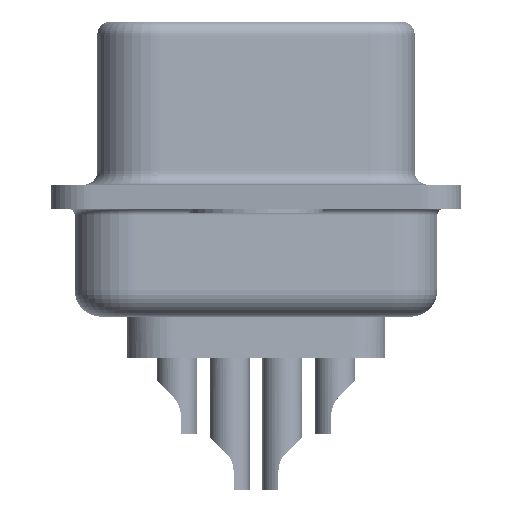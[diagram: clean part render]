
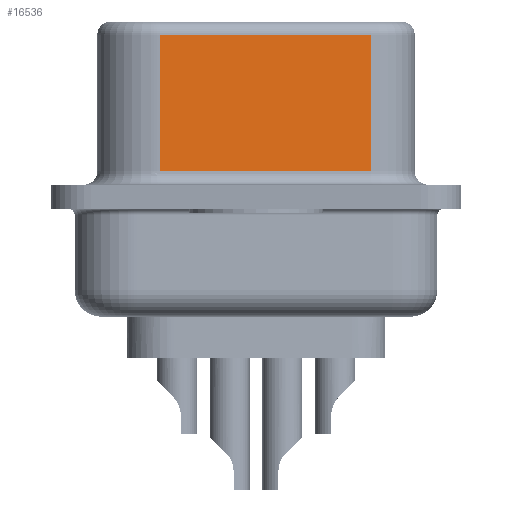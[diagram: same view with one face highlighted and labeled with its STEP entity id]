
A CAD part, left-side view. The second image highlights one B-rep face of the part: STEP entity #16536.
In plain terms, the highlighted planar face has unit normal (-0.985, -0.174, 0).
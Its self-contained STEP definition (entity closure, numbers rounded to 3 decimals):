
#374 = VECTOR ( 'NONE', #13509, 1000. ) ;
#705 = ORIENTED_EDGE ( 'NONE', *, *, #27809, .F. ) ;
#1121 = CARTESIAN_POINT ( 'NONE',  ( 5.128, -4.297, 0.95 ) ) ;
#1655 = EDGE_LOOP ( 'NONE', ( #705, #11699, #8295, #27172 ) ) ;
#2505 = CARTESIAN_POINT ( 'NONE',  ( 5.128, -4.297, 6.57 ) ) ;
#3045 = VERTEX_POINT ( 'NONE', #18886 ) ;
#3087 = VECTOR ( 'NONE', #18330, 1000. ) ;
#4540 = VECTOR ( 'NONE', #12022, 1000. ) ;
#5578 = CARTESIAN_POINT ( 'NONE',  ( 3.735, 3.603, 6.57 ) ) ;
#5744 = CARTESIAN_POINT ( 'NONE',  ( 5.128, -4.297, 0.95 ) ) ;
#8295 = ORIENTED_EDGE ( 'NONE', *, *, #33518, .T. ) ;
#8636 = EDGE_CURVE ( 'NONE', #32476, #25748, #24110, .T. ) ;
#10277 = CARTESIAN_POINT ( 'NONE',  ( 5.128, -4.297, 6.57 ) ) ;
#11154 = PLANE ( 'NONE',  #27211 ) ;
#11699 = ORIENTED_EDGE ( 'NONE', *, *, #22238, .T. ) ;
#12022 = DIRECTION ( 'NONE',  ( 0., 0., -1. ) ) ;
#12482 = LINE ( 'NONE', #33876, #3087 ) ;
#13314 = CARTESIAN_POINT ( 'NONE',  ( 3.735, 3.603, 0.95 ) ) ;
#13509 = DIRECTION ( 'NONE',  ( 0., 0., -1. ) ) ;
#16536 = ADVANCED_FACE ( 'NONE', ( #23476 ), #11154, .F. ) ;
#18330 = DIRECTION ( 'NONE',  ( -0.174, 0.985, 0. ) ) ;
#18831 = CARTESIAN_POINT ( 'NONE',  ( 5.128, -4.297, 6.07 ) ) ;
#18886 = CARTESIAN_POINT ( 'NONE',  ( 3.735, 3.603, 6.07 ) ) ;
#20629 = DIRECTION ( 'NONE',  ( -0.174, 0.985, 0. ) ) ;
#22238 = EDGE_CURVE ( 'NONE', #30195, #3045, #12482, .T. ) ;
#23476 = FACE_OUTER_BOUND ( 'NONE', #1655, .T. ) ;
#24110 = LINE ( 'NONE', #5744, #39064 ) ;
#25748 = VERTEX_POINT ( 'NONE', #1121 ) ;
#26689 = DIRECTION ( 'NONE',  ( 0.985, 0.174, 0. ) ) ;
#27172 = ORIENTED_EDGE ( 'NONE', *, *, #8636, .T. ) ;
#27211 = AXIS2_PLACEMENT_3D ( 'NONE', #2505, #26689, #20629 ) ;
#27809 = EDGE_CURVE ( 'NONE', #30195, #25748, #31260, .T. ) ;
#30195 = VERTEX_POINT ( 'NONE', #18831 ) ;
#31260 = LINE ( 'NONE', #10277, #374 ) ;
#32476 = VERTEX_POINT ( 'NONE', #13314 ) ;
#33518 = EDGE_CURVE ( 'NONE', #3045, #32476, #39640, .T. ) ;
#33876 = CARTESIAN_POINT ( 'NONE',  ( 5.128, -4.297, 6.07 ) ) ;
#39064 = VECTOR ( 'NONE', #39219, 1000. ) ;
#39219 = DIRECTION ( 'NONE',  ( 0.174, -0.985, 0. ) ) ;
#39640 = LINE ( 'NONE', #5578, #4540 ) ;
